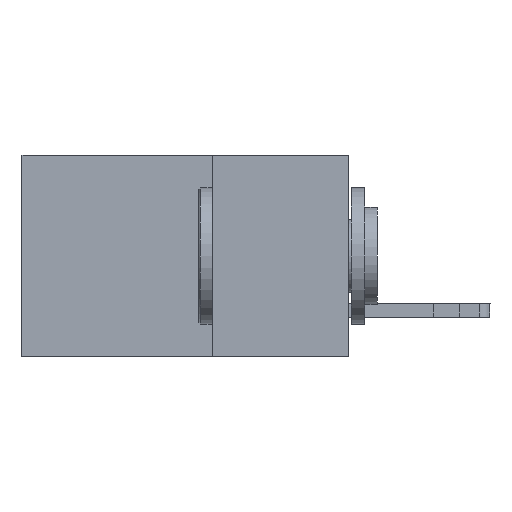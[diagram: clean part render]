
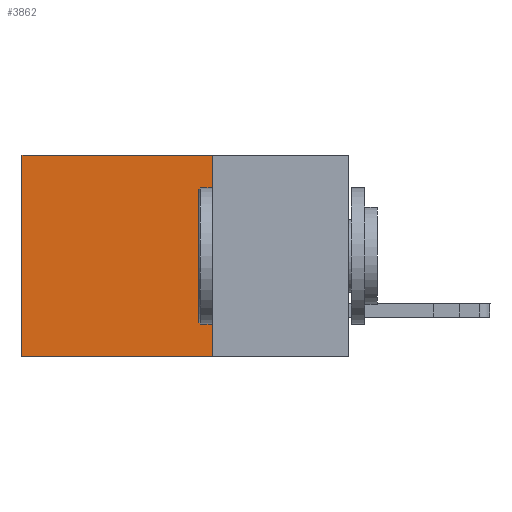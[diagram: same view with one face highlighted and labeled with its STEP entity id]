
A CAD part, left-side view. The second image highlights one B-rep face of the part: STEP entity #3862.
In plain terms, the highlighted planar face has unit normal (-1, 0, 0).
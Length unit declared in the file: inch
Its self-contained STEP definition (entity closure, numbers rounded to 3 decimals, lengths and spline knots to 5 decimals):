
#75 = DIRECTION ( 'NONE',  ( 0., 0., -1. ) ) ;
#1428 = EDGE_CURVE ( 'NONE', #12509, #10556, #3293, .T. ) ;
#1650 = ORIENTED_EDGE ( 'NONE', *, *, #16071, .F. ) ;
#1827 = PLANE ( 'NONE',  #10765 ) ;
#3293 = LINE ( 'NONE', #14405, #5145 ) ;
#3316 = CARTESIAN_POINT ( 'NONE',  ( 0.298, 0.6, 0. ) ) ;
#3779 = VERTEX_POINT ( 'NONE', #16934 ) ;
#3862 = ADVANCED_FACE ( 'NONE', ( #7346 ), #1827, .F. ) ;
#4550 = ORIENTED_EDGE ( 'NONE', *, *, #4699, .T. ) ;
#4699 = EDGE_CURVE ( 'NONE', #10556, #7355, #16797, .T. ) ;
#5145 = VECTOR ( 'NONE', #17148, 39.37008 ) ;
#5790 = CARTESIAN_POINT ( 'NONE',  ( 0.298, 0.6, 0. ) ) ;
#5830 = LINE ( 'NONE', #5914, #6378 ) ;
#5914 = CARTESIAN_POINT ( 'NONE',  ( 0.298, 0.25, -0.37 ) ) ;
#6378 = VECTOR ( 'NONE', #11380, 39.37008 ) ;
#7346 = FACE_OUTER_BOUND ( 'NONE', #16412, .T. ) ;
#7355 = VERTEX_POINT ( 'NONE', #11810 ) ;
#8517 = DIRECTION ( 'NONE',  ( 1., 0., 0. ) ) ;
#8606 = DIRECTION ( 'NONE',  ( 0., 0., -1. ) ) ;
#8652 = VECTOR ( 'NONE', #11365, 39.37008 ) ;
#10556 = VERTEX_POINT ( 'NONE', #3316 ) ;
#10765 = AXIS2_PLACEMENT_3D ( 'NONE', #11382, #8517, #8606 ) ;
#10901 = CARTESIAN_POINT ( 'NONE',  ( 0.298, 0.25, 0. ) ) ;
#11189 = LINE ( 'NONE', #15147, #8652 ) ;
#11347 = ORIENTED_EDGE ( 'NONE', *, *, #12232, .F. ) ;
#11365 = DIRECTION ( 'NONE',  ( 0., 0., -1. ) ) ;
#11380 = DIRECTION ( 'NONE',  ( 0., 1., 0. ) ) ;
#11382 = CARTESIAN_POINT ( 'NONE',  ( 0.298, 0.25, 0. ) ) ;
#11810 = CARTESIAN_POINT ( 'NONE',  ( 0.298, 0.6, -0.37 ) ) ;
#12232 = EDGE_CURVE ( 'NONE', #12509, #3779, #11189, .T. ) ;
#12509 = VERTEX_POINT ( 'NONE', #10901 ) ;
#14405 = CARTESIAN_POINT ( 'NONE',  ( 0.298, 0.25, 0. ) ) ;
#15147 = CARTESIAN_POINT ( 'NONE',  ( 0.298, 0.25, 0. ) ) ;
#16071 = EDGE_CURVE ( 'NONE', #3779, #7355, #5830, .T. ) ;
#16135 = ORIENTED_EDGE ( 'NONE', *, *, #1428, .T. ) ;
#16412 = EDGE_LOOP ( 'NONE', ( #4550, #1650, #11347, #16135 ) ) ;
#16507 = VECTOR ( 'NONE', #75, 39.37008 ) ;
#16797 = LINE ( 'NONE', #5790, #16507 ) ;
#16934 = CARTESIAN_POINT ( 'NONE',  ( 0.298, 0.25, -0.37 ) ) ;
#17148 = DIRECTION ( 'NONE',  ( 0., 1., 0. ) ) ;
